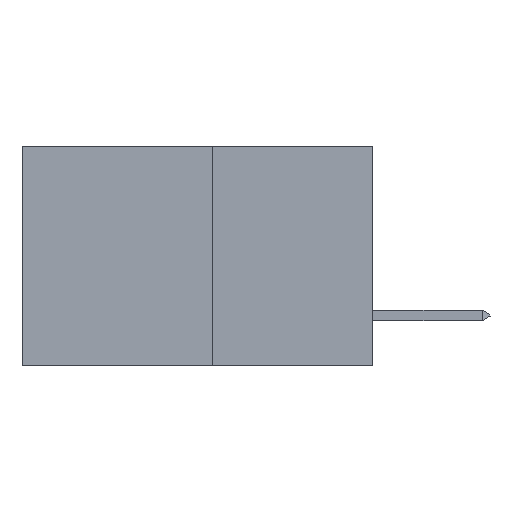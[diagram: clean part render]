
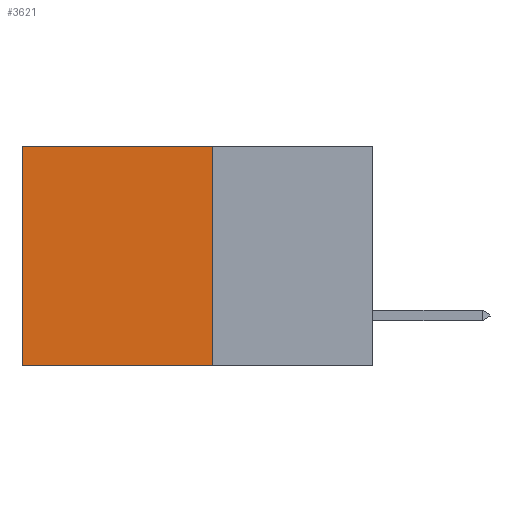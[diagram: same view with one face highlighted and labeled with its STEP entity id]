
A CAD part, left-side view. The second image highlights one B-rep face of the part: STEP entity #3621.
In plain terms, the highlighted planar face has unit normal (-1, 0, 0).
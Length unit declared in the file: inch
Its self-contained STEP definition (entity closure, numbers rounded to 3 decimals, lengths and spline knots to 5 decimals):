
#1415 = VECTOR ( 'NONE', #7203, 39.37008 ) ;
#1558 = ORIENTED_EDGE ( 'NONE', *, *, #1664, .T. ) ;
#1664 = EDGE_CURVE ( 'NONE', #5214, #5113, #4766, .T. ) ;
#2310 = LINE ( 'NONE', #7109, #12808 ) ;
#2448 = CARTESIAN_POINT ( 'NONE',  ( 0.277, 0.59, -0.37 ) ) ;
#3075 = CARTESIAN_POINT ( 'NONE',  ( 0.277, 0.27, -0.37 ) ) ;
#3340 = AXIS2_PLACEMENT_3D ( 'NONE', #10439, #10421, #10406 ) ;
#3621 = ADVANCED_FACE ( 'NONE', ( #10065 ), #10473, .F. ) ;
#3968 = EDGE_LOOP ( 'NONE', ( #1558, #6873, #9510, #12133 ) ) ;
#4112 = LINE ( 'NONE', #7633, #1415 ) ;
#4766 = LINE ( 'NONE', #11074, #7087 ) ;
#4905 = EDGE_CURVE ( 'NONE', #8557, #5113, #4112, .T. ) ;
#5113 = VERTEX_POINT ( 'NONE', #2448 ) ;
#5214 = VERTEX_POINT ( 'NONE', #12741 ) ;
#6873 = ORIENTED_EDGE ( 'NONE', *, *, #4905, .F. ) ;
#7087 = VECTOR ( 'NONE', #10705, 39.37008 ) ;
#7109 = CARTESIAN_POINT ( 'NONE',  ( 0.277, 0.27, 0. ) ) ;
#7134 = LINE ( 'NONE', #12879, #9761 ) ;
#7203 = DIRECTION ( 'NONE',  ( 0., 1., 0. ) ) ;
#7538 = EDGE_CURVE ( 'NONE', #12443, #8557, #7134, .T. ) ;
#7633 = CARTESIAN_POINT ( 'NONE',  ( 0.277, 0.27, -0.37 ) ) ;
#8557 = VERTEX_POINT ( 'NONE', #3075 ) ;
#8993 = DIRECTION ( 'NONE',  ( 0., 0., -1. ) ) ;
#9510 = ORIENTED_EDGE ( 'NONE', *, *, #7538, .F. ) ;
#9761 = VECTOR ( 'NONE', #8993, 39.37008 ) ;
#10065 = FACE_OUTER_BOUND ( 'NONE', #3968, .T. ) ;
#10406 = DIRECTION ( 'NONE',  ( 0., 0., -1. ) ) ;
#10421 = DIRECTION ( 'NONE',  ( 1., 0., 0. ) ) ;
#10439 = CARTESIAN_POINT ( 'NONE',  ( 0.277, 0.27, -0.37 ) ) ;
#10473 = PLANE ( 'NONE',  #3340 ) ;
#10705 = DIRECTION ( 'NONE',  ( 0., 0., -1. ) ) ;
#10776 = CARTESIAN_POINT ( 'NONE',  ( 0.277, 0.27, 0. ) ) ;
#11074 = CARTESIAN_POINT ( 'NONE',  ( 0.277, 0.59, -0.37 ) ) ;
#12025 = DIRECTION ( 'NONE',  ( 0., 1., 0. ) ) ;
#12133 = ORIENTED_EDGE ( 'NONE', *, *, #12689, .T. ) ;
#12443 = VERTEX_POINT ( 'NONE', #10776 ) ;
#12689 = EDGE_CURVE ( 'NONE', #12443, #5214, #2310, .T. ) ;
#12741 = CARTESIAN_POINT ( 'NONE',  ( 0.277, 0.59, 0. ) ) ;
#12808 = VECTOR ( 'NONE', #12025, 39.37008 ) ;
#12879 = CARTESIAN_POINT ( 'NONE',  ( 0.277, 0.27, -0.37 ) ) ;
